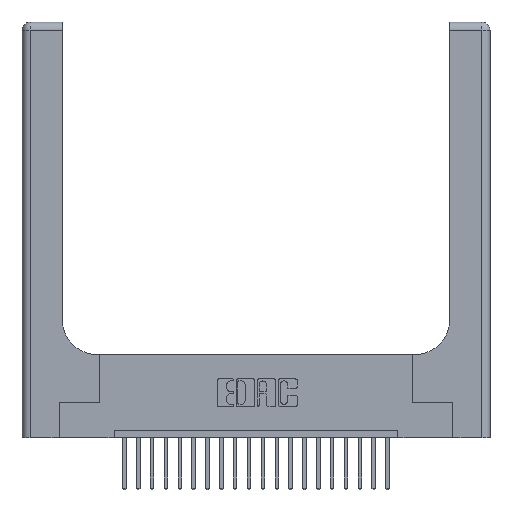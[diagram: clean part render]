
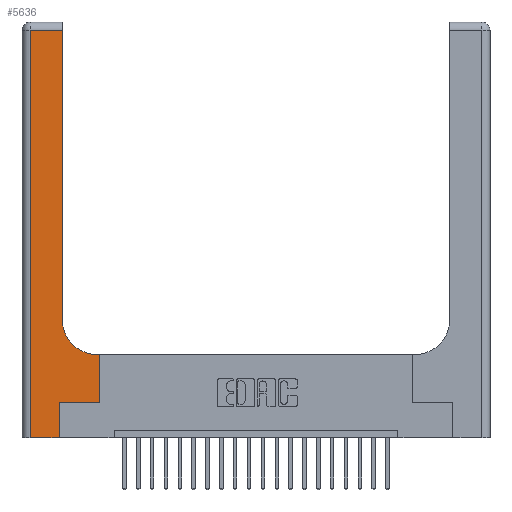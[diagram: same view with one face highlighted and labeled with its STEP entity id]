
A CAD part, top view. The second image highlights one B-rep face of the part: STEP entity #5636.
In plain terms, the highlighted planar face has unit normal (0, 0, 1).
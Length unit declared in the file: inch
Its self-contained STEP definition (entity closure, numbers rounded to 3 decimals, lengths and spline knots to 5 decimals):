
#103 = ORIENTED_EDGE ( 'NONE', *, *, #9656, .T. ) ;
#402 = DIRECTION ( 'NONE',  ( -1., 0., 0. ) ) ;
#890 = DIRECTION ( 'NONE',  ( -1., 0., 0. ) ) ;
#954 = CIRCLE ( 'NONE', #1272, 0.25 ) ;
#1006 = CARTESIAN_POINT ( 'NONE',  ( 0.269, 0.25, 0.37 ) ) ;
#1124 = CARTESIAN_POINT ( 'NONE',  ( 0.2915, 0.6, 0.37 ) ) ;
#1272 = AXIS2_PLACEMENT_3D ( 'NONE', #17686, #8727, #5444 ) ;
#1912 = LINE ( 'NONE', #17853, #8856 ) ;
#2077 = VERTEX_POINT ( 'NONE', #22727 ) ;
#2285 = ORIENTED_EDGE ( 'NONE', *, *, #20513, .T. ) ;
#2419 = LINE ( 'NONE', #4808, #4922 ) ;
#2609 = VECTOR ( 'NONE', #9465, 39.37008 ) ;
#2674 = VECTOR ( 'NONE', #22249, 39.37008 ) ;
#3403 = CARTESIAN_POINT ( 'NONE',  ( 0., 3., 0.37 ) ) ;
#4351 = LINE ( 'NONE', #20302, #15258 ) ;
#4617 = LINE ( 'NONE', #1006, #2674 ) ;
#4808 = CARTESIAN_POINT ( 'NONE',  ( 0.269, 0., 0.37 ) ) ;
#4922 = VECTOR ( 'NONE', #10272, 39.37008 ) ;
#5392 = VERTEX_POINT ( 'NONE', #19287 ) ;
#5444 = DIRECTION ( 'NONE',  ( 1., 0., 0. ) ) ;
#5632 = VECTOR ( 'NONE', #890, 39.37008 ) ;
#5636 = ADVANCED_FACE ( 'NONE', ( #20467 ), #22940, .F. ) ;
#6306 = DIRECTION ( 'NONE',  ( 0., 1., 0. ) ) ;
#6477 = VERTEX_POINT ( 'NONE', #14988 ) ;
#8193 = CARTESIAN_POINT ( 'NONE',  ( 0.5585, 0.6, 0.37 ) ) ;
#8439 = VECTOR ( 'NONE', #21450, 39.37008 ) ;
#8727 = DIRECTION ( 'NONE',  ( 0., 0., -1. ) ) ;
#8856 = VECTOR ( 'NONE', #8881, 39.37008 ) ;
#8861 = CARTESIAN_POINT ( 'NONE',  ( 0.2915, 3., 0.37 ) ) ;
#8881 = DIRECTION ( 'NONE',  ( 1., 0., 0. ) ) ;
#8938 = VERTEX_POINT ( 'NONE', #8193 ) ;
#9465 = DIRECTION ( 'NONE',  ( -1., 0., 0. ) ) ;
#9656 = EDGE_CURVE ( 'NONE', #6477, #10675, #954, .T. ) ;
#10272 = DIRECTION ( 'NONE',  ( 0., 1., 0. ) ) ;
#10287 = ORIENTED_EDGE ( 'NONE', *, *, #18494, .T. ) ;
#10597 = CARTESIAN_POINT ( 'NONE',  ( 0.2915, 0.85, 0.37 ) ) ;
#10675 = VERTEX_POINT ( 'NONE', #10597 ) ;
#10977 = CARTESIAN_POINT ( 'NONE',  ( 0., 2.94, 0.37 ) ) ;
#11161 = CARTESIAN_POINT ( 'NONE',  ( 0.5585, 0.25, 0.37 ) ) ;
#12127 = VERTEX_POINT ( 'NONE', #21830 ) ;
#12198 = VERTEX_POINT ( 'NONE', #11161 ) ;
#12604 = ORIENTED_EDGE ( 'NONE', *, *, #14180, .T. ) ;
#12663 = LINE ( 'NONE', #1124, #5632 ) ;
#13090 = CARTESIAN_POINT ( 'NONE',  ( 0.06, 2.94, 0.37 ) ) ;
#13396 = DIRECTION ( 'NONE',  ( 0., -1., 0. ) ) ;
#13545 = LINE ( 'NONE', #22399, #17168 ) ;
#13724 = EDGE_LOOP ( 'NONE', ( #12604, #17733, #2285, #18970, #10287, #14351, #15661, #17915, #103 ) ) ;
#13975 = EDGE_CURVE ( 'NONE', #12198, #8938, #13545, .T. ) ;
#14180 = EDGE_CURVE ( 'NONE', #10675, #12127, #18017, .T. ) ;
#14230 = CARTESIAN_POINT ( 'NONE',  ( 0.06, 0., 0.37 ) ) ;
#14351 = ORIENTED_EDGE ( 'NONE', *, *, #20612, .T. ) ;
#14643 = EDGE_CURVE ( 'NONE', #8938, #6477, #12663, .T. ) ;
#14988 = CARTESIAN_POINT ( 'NONE',  ( 0.5415, 0.6, 0.37 ) ) ;
#15258 = VECTOR ( 'NONE', #13396, 39.37008 ) ;
#15661 = ORIENTED_EDGE ( 'NONE', *, *, #13975, .T. ) ;
#16215 = AXIS2_PLACEMENT_3D ( 'NONE', #3403, #18213, #402 ) ;
#16692 = VERTEX_POINT ( 'NONE', #14230 ) ;
#17168 = VECTOR ( 'NONE', #6306, 39.37008 ) ;
#17683 = VERTEX_POINT ( 'NONE', #13090 ) ;
#17686 = CARTESIAN_POINT ( 'NONE',  ( 0.5415, 0.85, 0.37 ) ) ;
#17733 = ORIENTED_EDGE ( 'NONE', *, *, #21671, .T. ) ;
#17853 = CARTESIAN_POINT ( 'NONE',  ( 0., 0., 0.37 ) ) ;
#17894 = EDGE_CURVE ( 'NONE', #16692, #2077, #1912, .T. ) ;
#17915 = ORIENTED_EDGE ( 'NONE', *, *, #14643, .T. ) ;
#18017 = LINE ( 'NONE', #8861, #8439 ) ;
#18213 = DIRECTION ( 'NONE',  ( 0., 0., -1. ) ) ;
#18494 = EDGE_CURVE ( 'NONE', #2077, #5392, #2419, .T. ) ;
#18970 = ORIENTED_EDGE ( 'NONE', *, *, #17894, .T. ) ;
#19287 = CARTESIAN_POINT ( 'NONE',  ( 0.269, 0.25, 0.37 ) ) ;
#20302 = CARTESIAN_POINT ( 'NONE',  ( 0.06, 3., 0.37 ) ) ;
#20467 = FACE_OUTER_BOUND ( 'NONE', #13724, .T. ) ;
#20513 = EDGE_CURVE ( 'NONE', #17683, #16692, #4351, .T. ) ;
#20612 = EDGE_CURVE ( 'NONE', #5392, #12198, #4617, .T. ) ;
#20828 = LINE ( 'NONE', #10977, #2609 ) ;
#21450 = DIRECTION ( 'NONE',  ( 0., 1., 0. ) ) ;
#21671 = EDGE_CURVE ( 'NONE', #12127, #17683, #20828, .T. ) ;
#21830 = CARTESIAN_POINT ( 'NONE',  ( 0.2915, 2.94, 0.37 ) ) ;
#22249 = DIRECTION ( 'NONE',  ( 1., 0., 0. ) ) ;
#22399 = CARTESIAN_POINT ( 'NONE',  ( 0.5585, 0.25, 0.37 ) ) ;
#22727 = CARTESIAN_POINT ( 'NONE',  ( 0.269, 0., 0.37 ) ) ;
#22940 = PLANE ( 'NONE',  #16215 ) ;
